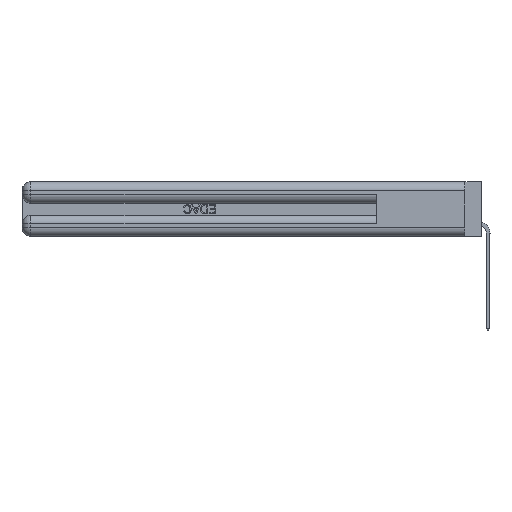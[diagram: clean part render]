
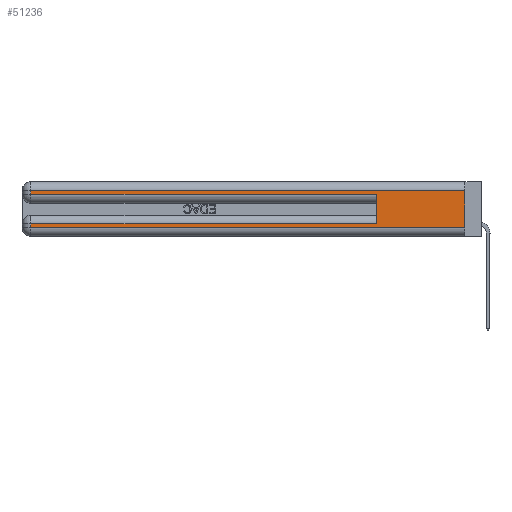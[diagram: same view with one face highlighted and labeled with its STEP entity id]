
A CAD part, left-side view. The second image highlights one B-rep face of the part: STEP entity #51236.
In plain terms, the highlighted planar face has unit normal (-1, 0, 0).
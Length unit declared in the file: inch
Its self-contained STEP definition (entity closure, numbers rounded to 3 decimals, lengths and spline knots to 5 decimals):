
#1533 = DIRECTION ( 'NONE',  ( 0., 1., 0. ) ) ;
#2323 = DIRECTION ( 'NONE',  ( 0., 0., -1. ) ) ;
#2446 = VECTOR ( 'NONE', #47025, 39.37008 ) ;
#2890 = LINE ( 'NONE', #26884, #12901 ) ;
#2902 = CARTESIAN_POINT ( 'NONE',  ( 0., 2.94, 0.06 ) ) ;
#3077 = FACE_OUTER_BOUND ( 'NONE', #48710, .T. ) ;
#4710 = DIRECTION ( 'NONE',  ( 0., 0., -1. ) ) ;
#4856 = CARTESIAN_POINT ( 'NONE',  ( 0., 0.6, 0.085 ) ) ;
#6058 = EDGE_CURVE ( 'NONE', #13317, #47795, #29490, .T. ) ;
#9018 = VERTEX_POINT ( 'NONE', #2902 ) ;
#9172 = EDGE_CURVE ( 'NONE', #27797, #47540, #50395, .T. ) ;
#10922 = PLANE ( 'NONE',  #33239 ) ;
#11572 = EDGE_CURVE ( 'NONE', #27797, #42275, #24201, .T. ) ;
#12901 = VECTOR ( 'NONE', #39673, 39.37008 ) ;
#13317 = VERTEX_POINT ( 'NONE', #4856 ) ;
#16071 = VERTEX_POINT ( 'NONE', #54740 ) ;
#16128 = DIRECTION ( 'NONE',  ( 0., 1., 0. ) ) ;
#18275 = DIRECTION ( 'NONE',  ( 0., 0., -1. ) ) ;
#18470 = CARTESIAN_POINT ( 'NONE',  ( 0., 0., 0.31 ) ) ;
#20584 = CARTESIAN_POINT ( 'NONE',  ( 0., 0., 0.06 ) ) ;
#24201 = LINE ( 'NONE', #18470, #31395 ) ;
#24922 = VECTOR ( 'NONE', #4710, 39.37008 ) ;
#26407 = VECTOR ( 'NONE', #2323, 39.37008 ) ;
#26884 = CARTESIAN_POINT ( 'NONE',  ( 0., 0., 0.285 ) ) ;
#27797 = VERTEX_POINT ( 'NONE', #34710 ) ;
#29221 = ORIENTED_EDGE ( 'NONE', *, *, #41423, .F. ) ;
#29490 = LINE ( 'NONE', #48700, #40031 ) ;
#31395 = VECTOR ( 'NONE', #1533, 39.37008 ) ;
#31744 = DIRECTION ( 'NONE',  ( 1., 0., 0. ) ) ;
#32746 = DIRECTION ( 'NONE',  ( 0., -1., 0. ) ) ;
#33232 = LINE ( 'NONE', #43479, #49861 ) ;
#33239 = AXIS2_PLACEMENT_3D ( 'NONE', #44784, #31744, #49245 ) ;
#34314 = EDGE_CURVE ( 'NONE', #39969, #16071, #2890, .T. ) ;
#34710 = CARTESIAN_POINT ( 'NONE',  ( 0., 0., 0.31 ) ) ;
#36108 = LINE ( 'NONE', #37003, #24922 ) ;
#37003 = CARTESIAN_POINT ( 'NONE',  ( 0., 2.94, 0.37 ) ) ;
#38596 = ORIENTED_EDGE ( 'NONE', *, *, #47313, .T. ) ;
#39125 = CARTESIAN_POINT ( 'NONE',  ( 0., 0., 0.06 ) ) ;
#39673 = DIRECTION ( 'NONE',  ( 0., -1., 0. ) ) ;
#39969 = VERTEX_POINT ( 'NONE', #41679 ) ;
#39990 = ORIENTED_EDGE ( 'NONE', *, *, #11572, .T. ) ;
#40031 = VECTOR ( 'NONE', #16128, 39.37008 ) ;
#40483 = ORIENTED_EDGE ( 'NONE', *, *, #9172, .F. ) ;
#40849 = CARTESIAN_POINT ( 'NONE',  ( 0., 0., 0.37 ) ) ;
#41423 = EDGE_CURVE ( 'NONE', #13317, #16071, #43536, .T. ) ;
#41679 = CARTESIAN_POINT ( 'NONE',  ( 0., 2.94, 0.285 ) ) ;
#42275 = VERTEX_POINT ( 'NONE', #47052 ) ;
#43479 = CARTESIAN_POINT ( 'NONE',  ( 0., 2.94, 0.37 ) ) ;
#43536 = LINE ( 'NONE', #51273, #2446 ) ;
#44524 = EDGE_CURVE ( 'NONE', #9018, #47540, #45090, .T. ) ;
#44784 = CARTESIAN_POINT ( 'NONE',  ( 0., 0., 0.37 ) ) ;
#45090 = LINE ( 'NONE', #20584, #49091 ) ;
#45422 = ORIENTED_EDGE ( 'NONE', *, *, #54450, .T. ) ;
#47025 = DIRECTION ( 'NONE',  ( 0., 0., 1. ) ) ;
#47052 = CARTESIAN_POINT ( 'NONE',  ( 0., 2.94, 0.31 ) ) ;
#47313 = EDGE_CURVE ( 'NONE', #42275, #39969, #36108, .T. ) ;
#47540 = VERTEX_POINT ( 'NONE', #39125 ) ;
#47795 = VERTEX_POINT ( 'NONE', #47948 ) ;
#47948 = CARTESIAN_POINT ( 'NONE',  ( 0., 2.94, 0.085 ) ) ;
#48700 = CARTESIAN_POINT ( 'NONE',  ( 0., 0., 0.085 ) ) ;
#48710 = EDGE_LOOP ( 'NONE', ( #40483, #39990, #38596, #53101, #29221, #52182, #45422, #49770 ) ) ;
#49091 = VECTOR ( 'NONE', #32746, 39.37008 ) ;
#49245 = DIRECTION ( 'NONE',  ( 0., 0., -1. ) ) ;
#49770 = ORIENTED_EDGE ( 'NONE', *, *, #44524, .T. ) ;
#49861 = VECTOR ( 'NONE', #18275, 39.37008 ) ;
#50395 = LINE ( 'NONE', #40849, #26407 ) ;
#51236 = ADVANCED_FACE ( 'NONE', ( #3077 ), #10922, .F. ) ;
#51273 = CARTESIAN_POINT ( 'NONE',  ( 0., 0.6, 0.145 ) ) ;
#52182 = ORIENTED_EDGE ( 'NONE', *, *, #6058, .T. ) ;
#53101 = ORIENTED_EDGE ( 'NONE', *, *, #34314, .T. ) ;
#54450 = EDGE_CURVE ( 'NONE', #47795, #9018, #33232, .T. ) ;
#54740 = CARTESIAN_POINT ( 'NONE',  ( 0., 0.6, 0.285 ) ) ;
